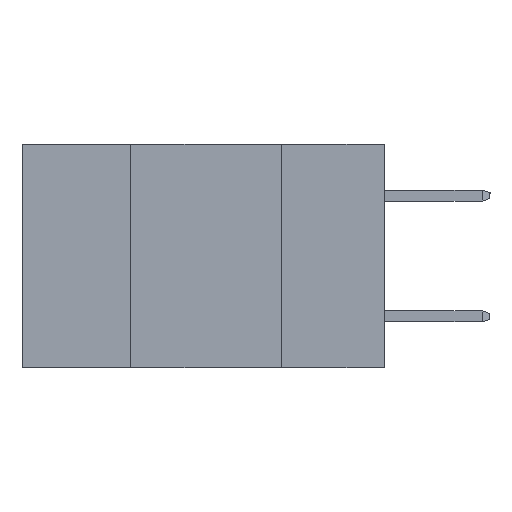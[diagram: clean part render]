
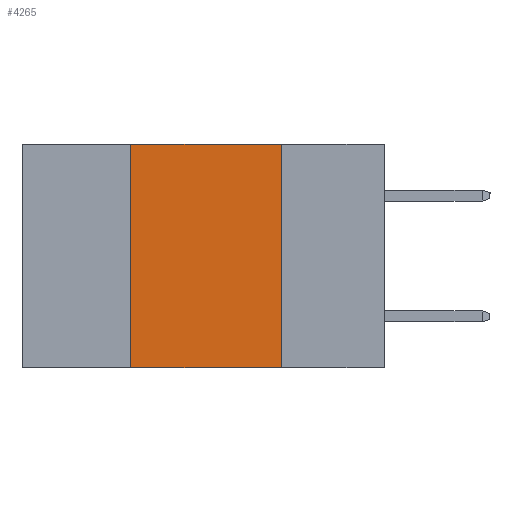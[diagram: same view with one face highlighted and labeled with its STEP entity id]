
A CAD part, left-side view. The second image highlights one B-rep face of the part: STEP entity #4265.
In plain terms, the highlighted planar face has unit normal (-1, 0, 0).
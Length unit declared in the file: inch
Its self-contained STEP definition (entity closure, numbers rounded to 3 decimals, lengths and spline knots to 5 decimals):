
#329 = CARTESIAN_POINT ( 'NONE',  ( 0., 0.6, 0. ) ) ;
#980 = ORIENTED_EDGE ( 'NONE', *, *, #8648, .T. ) ;
#1334 = DIRECTION ( 'NONE',  ( 0., 0., -1. ) ) ;
#2621 = AXIS2_PLACEMENT_3D ( 'NONE', #11695, #6974, #5970 ) ;
#3138 = VERTEX_POINT ( 'NONE', #15342 ) ;
#3329 = EDGE_CURVE ( 'NONE', #15299, #13061, #3984, .T. ) ;
#3698 = LINE ( 'NONE', #7235, #9886 ) ;
#3873 = EDGE_LOOP ( 'NONE', ( #4094, #14180, #4542, #980 ) ) ;
#3984 = LINE ( 'NONE', #7608, #5319 ) ;
#4094 = ORIENTED_EDGE ( 'NONE', *, *, #14996, .F. ) ;
#4265 = ADVANCED_FACE ( 'NONE', ( #6893 ), #9250, .F. ) ;
#4286 = CARTESIAN_POINT ( 'NONE',  ( 0., 0.42, -0.37 ) ) ;
#4542 = ORIENTED_EDGE ( 'NONE', *, *, #3329, .F. ) ;
#4835 = LINE ( 'NONE', #329, #15375 ) ;
#5319 = VECTOR ( 'NONE', #7526, 39.37008 ) ;
#5970 = DIRECTION ( 'NONE',  ( 0., 0., -1. ) ) ;
#5996 = VERTEX_POINT ( 'NONE', #9018 ) ;
#6893 = FACE_OUTER_BOUND ( 'NONE', #3873, .T. ) ;
#6974 = DIRECTION ( 'NONE',  ( 1., 0., 0. ) ) ;
#7235 = CARTESIAN_POINT ( 'NONE',  ( 0., 0.17, -0.37 ) ) ;
#7526 = DIRECTION ( 'NONE',  ( 0., 0., 1. ) ) ;
#7608 = CARTESIAN_POINT ( 'NONE',  ( 0., 0.42, -0.37 ) ) ;
#7789 = LINE ( 'NONE', #12450, #13906 ) ;
#8648 = EDGE_CURVE ( 'NONE', #15299, #3138, #7789, .T. ) ;
#9018 = CARTESIAN_POINT ( 'NONE',  ( 0., 0.17, 0. ) ) ;
#9250 = PLANE ( 'NONE',  #2621 ) ;
#9540 = DIRECTION ( 'NONE',  ( 0., -1., 0. ) ) ;
#9886 = VECTOR ( 'NONE', #1334, 39.37008 ) ;
#10294 = DIRECTION ( 'NONE',  ( 0., -1., 0. ) ) ;
#11695 = CARTESIAN_POINT ( 'NONE',  ( 0., 0.6, 0. ) ) ;
#12119 = CARTESIAN_POINT ( 'NONE',  ( 0., 0.42, 0. ) ) ;
#12450 = CARTESIAN_POINT ( 'NONE',  ( 0., 0.6, -0.37 ) ) ;
#13061 = VERTEX_POINT ( 'NONE', #12119 ) ;
#13906 = VECTOR ( 'NONE', #10294, 39.37008 ) ;
#14180 = ORIENTED_EDGE ( 'NONE', *, *, #14462, .F. ) ;
#14462 = EDGE_CURVE ( 'NONE', #13061, #5996, #4835, .T. ) ;
#14996 = EDGE_CURVE ( 'NONE', #5996, #3138, #3698, .T. ) ;
#15299 = VERTEX_POINT ( 'NONE', #4286 ) ;
#15342 = CARTESIAN_POINT ( 'NONE',  ( 0., 0.17, -0.37 ) ) ;
#15375 = VECTOR ( 'NONE', #9540, 39.37008 ) ;
